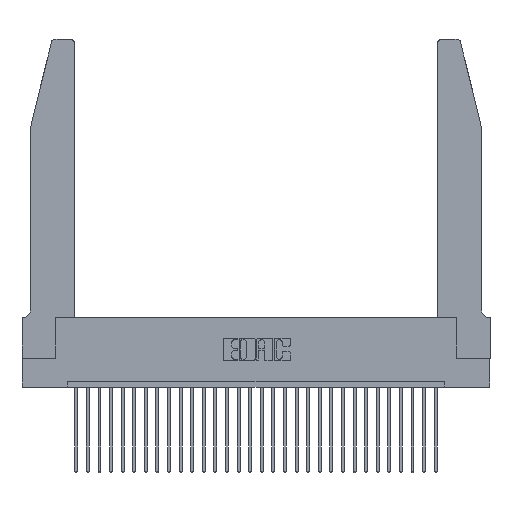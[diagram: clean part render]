
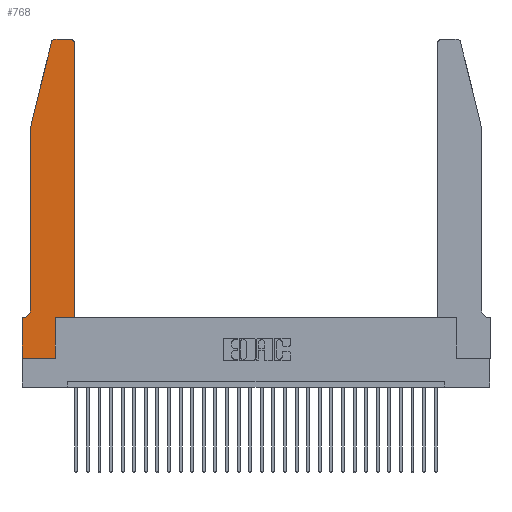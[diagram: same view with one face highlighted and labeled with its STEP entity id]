
A CAD part, top view. The second image highlights one B-rep face of the part: STEP entity #768.
In plain terms, the highlighted planar face has unit normal (0, 0, 1).
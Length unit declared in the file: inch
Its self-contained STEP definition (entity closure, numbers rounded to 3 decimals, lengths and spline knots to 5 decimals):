
#106 = CIRCLE ( 'NONE', #23955, 0.07 ) ;
#128 = CARTESIAN_POINT ( 'NONE',  ( 0.284, 2.72, 0.37 ) ) ;
#189 = CARTESIAN_POINT ( 'NONE',  ( 0., 0., 0.37 ) ) ;
#768 = ADVANCED_FACE ( 'NONE', ( #9896 ), #13526, .T. ) ;
#1057 = DIRECTION ( 'NONE',  ( -1., 0., 0. ) ) ;
#1212 = LINE ( 'NONE', #5877, #19064 ) ;
#1213 = CARTESIAN_POINT ( 'NONE',  ( 0.0755, 0.42, 0.37 ) ) ;
#1578 = EDGE_CURVE ( 'NONE', #16728, #28501, #26247, .T. ) ;
#1632 = CARTESIAN_POINT ( 'NONE',  ( 0.284, 2.75, 0.37 ) ) ;
#1847 = ORIENTED_EDGE ( 'NONE', *, *, #1578, .T. ) ;
#2159 = CARTESIAN_POINT ( 'NONE',  ( 0., 0., 0.37 ) ) ;
#2677 = EDGE_CURVE ( 'NONE', #13894, #16933, #22546, .T. ) ;
#2738 = EDGE_CURVE ( 'NONE', #5815, #26212, #29479, .T. ) ;
#3131 = DIRECTION ( 'NONE',  ( 1., 0., 0. ) ) ;
#3536 = VERTEX_POINT ( 'NONE', #14159 ) ;
#4017 = LINE ( 'NONE', #13214, #9822 ) ;
#4064 = VECTOR ( 'NONE', #15547, 39.37008 ) ;
#4070 = DIRECTION ( 'NONE',  ( 0., -1., 0. ) ) ;
#4321 = VERTEX_POINT ( 'NONE', #14307 ) ;
#5070 = CARTESIAN_POINT ( 'NONE',  ( 0.2865, 0.35, 0.37 ) ) ;
#5147 = ORIENTED_EDGE ( 'NONE', *, *, #2677, .T. ) ;
#5507 = LINE ( 'NONE', #17265, #9161 ) ;
#5815 = VERTEX_POINT ( 'NONE', #24547 ) ;
#5848 = VERTEX_POINT ( 'NONE', #1213 ) ;
#5851 = LINE ( 'NONE', #25435, #27350 ) ;
#5877 = CARTESIAN_POINT ( 'NONE',  ( 0.4505, 0.35, 0.37 ) ) ;
#5879 = AXIS2_PLACEMENT_3D ( 'NONE', #23144, #23545, #6950 ) ;
#5939 = CARTESIAN_POINT ( 'NONE',  ( 0.2865, 0., 0.37 ) ) ;
#6080 = ORIENTED_EDGE ( 'NONE', *, *, #2738, .T. ) ;
#6813 = DIRECTION ( 'NONE',  ( 1., 0., 0. ) ) ;
#6950 = DIRECTION ( 'NONE',  ( 1., 0., 0. ) ) ;
#7384 = EDGE_CURVE ( 'NONE', #10901, #3536, #1212, .T. ) ;
#7541 = ORIENTED_EDGE ( 'NONE', *, *, #28936, .T. ) ;
#8849 = EDGE_CURVE ( 'NONE', #28679, #5815, #5851, .T. ) ;
#9161 = VECTOR ( 'NONE', #3131, 39.37008 ) ;
#9822 = VECTOR ( 'NONE', #4070, 39.37008 ) ;
#9896 = FACE_OUTER_BOUND ( 'NONE', #27709, .T. ) ;
#10157 = VECTOR ( 'NONE', #23040, 39.37008 ) ;
#10209 = ORIENTED_EDGE ( 'NONE', *, *, #8849, .T. ) ;
#10570 = DIRECTION ( 'NONE',  ( 0., 1., 0. ) ) ;
#10901 = VERTEX_POINT ( 'NONE', #24233 ) ;
#10965 = ORIENTED_EDGE ( 'NONE', *, *, #25622, .T. ) ;
#10980 = CARTESIAN_POINT ( 'NONE',  ( 0.2605, 2.75, 0.37 ) ) ;
#11596 = EDGE_CURVE ( 'NONE', #5848, #28679, #106, .T. ) ;
#11744 = DIRECTION ( 'NONE',  ( 0., 0., 1. ) ) ;
#12135 = ORIENTED_EDGE ( 'NONE', *, *, #24043, .T. ) ;
#12158 = DIRECTION ( 'NONE',  ( -0.239, -0.971, 0. ) ) ;
#13214 = CARTESIAN_POINT ( 'NONE',  ( 0.0755, 2., 0.37 ) ) ;
#13310 = EDGE_CURVE ( 'NONE', #26212, #16728, #5507, .T. ) ;
#13526 = PLANE ( 'NONE',  #18339 ) ;
#13565 = DIRECTION ( 'NONE',  ( 1., 0., 0. ) ) ;
#13894 = VERTEX_POINT ( 'NONE', #26932 ) ;
#14159 = CARTESIAN_POINT ( 'NONE',  ( 0.4505, 2.72, 0.37 ) ) ;
#14307 = CARTESIAN_POINT ( 'NONE',  ( 0.0755, 2., 0.37 ) ) ;
#14521 = VECTOR ( 'NONE', #29889, 39.37008 ) ;
#15547 = DIRECTION ( 'NONE',  ( 0., 1., 0. ) ) ;
#15775 = VECTOR ( 'NONE', #12158, 39.37008 ) ;
#16141 = LINE ( 'NONE', #19104, #15775 ) ;
#16728 = VERTEX_POINT ( 'NONE', #5939 ) ;
#16933 = VERTEX_POINT ( 'NONE', #1632 ) ;
#17066 = CARTESIAN_POINT ( 'NONE',  ( 0.0055, 0.35, 0.37 ) ) ;
#17265 = CARTESIAN_POINT ( 'NONE',  ( 0., 0., 0.37 ) ) ;
#17342 = ORIENTED_EDGE ( 'NONE', *, *, #13310, .T. ) ;
#18001 = CARTESIAN_POINT ( 'NONE',  ( 0.2865, 0.35, 0.37 ) ) ;
#18339 = AXIS2_PLACEMENT_3D ( 'NONE', #25265, #20676, #6813 ) ;
#18994 = DIRECTION ( 'NONE',  ( 1., 0., 0. ) ) ;
#19064 = VECTOR ( 'NONE', #10570, 39.37008 ) ;
#19104 = CARTESIAN_POINT ( 'NONE',  ( 0.0755, 2., 0.37 ) ) ;
#19970 = ORIENTED_EDGE ( 'NONE', *, *, #11596, .T. ) ;
#20562 = DIRECTION ( 'NONE',  ( -1., 0., 0. ) ) ;
#20676 = DIRECTION ( 'NONE',  ( 0., 0., 1. ) ) ;
#20986 = LINE ( 'NONE', #27531, #26843 ) ;
#22546 = LINE ( 'NONE', #10980, #14521 ) ;
#22591 = CIRCLE ( 'NONE', #5879, 0.03 ) ;
#22804 = CARTESIAN_POINT ( 'NONE',  ( 0.25487, 2.72718, 0.37 ) ) ;
#23040 = DIRECTION ( 'NONE',  ( 0., -1., 0. ) ) ;
#23144 = CARTESIAN_POINT ( 'NONE',  ( 0.4205, 2.72, 0.37 ) ) ;
#23246 = AXIS2_PLACEMENT_3D ( 'NONE', #128, #11744, #18994 ) ;
#23545 = DIRECTION ( 'NONE',  ( 0., 0., 1. ) ) ;
#23955 = AXIS2_PLACEMENT_3D ( 'NONE', #26859, #24709, #1057 ) ;
#24043 = EDGE_CURVE ( 'NONE', #4321, #5848, #4017, .T. ) ;
#24112 = VERTEX_POINT ( 'NONE', #22804 ) ;
#24197 = ORIENTED_EDGE ( 'NONE', *, *, #26072, .T. ) ;
#24233 = CARTESIAN_POINT ( 'NONE',  ( 0.4505, 0.35, 0.37 ) ) ;
#24247 = EDGE_CURVE ( 'NONE', #3536, #13894, #22591, .T. ) ;
#24547 = CARTESIAN_POINT ( 'NONE',  ( 0., 0.35, 0.37 ) ) ;
#24709 = DIRECTION ( 'NONE',  ( 0., 0., -1. ) ) ;
#25265 = CARTESIAN_POINT ( 'NONE',  ( 0., 0.35, 0.37 ) ) ;
#25435 = CARTESIAN_POINT ( 'NONE',  ( 0.0755, 0.35, 0.37 ) ) ;
#25622 = EDGE_CURVE ( 'NONE', #16933, #24112, #29752, .T. ) ;
#25937 = ORIENTED_EDGE ( 'NONE', *, *, #24247, .T. ) ;
#26072 = EDGE_CURVE ( 'NONE', #28501, #10901, #20986, .T. ) ;
#26212 = VERTEX_POINT ( 'NONE', #189 ) ;
#26247 = LINE ( 'NONE', #18001, #4064 ) ;
#26843 = VECTOR ( 'NONE', #13565, 39.37008 ) ;
#26859 = CARTESIAN_POINT ( 'NONE',  ( 0.0055, 0.42, 0.37 ) ) ;
#26932 = CARTESIAN_POINT ( 'NONE',  ( 0.4205, 2.75, 0.37 ) ) ;
#27350 = VECTOR ( 'NONE', #20562, 39.37008 ) ;
#27531 = CARTESIAN_POINT ( 'NONE',  ( 0.4505, 0.35, 0.37 ) ) ;
#27709 = EDGE_LOOP ( 'NONE', ( #5147, #10965, #7541, #12135, #19970, #10209, #6080, #17342, #1847, #24197, #28834, #25937 ) ) ;
#28501 = VERTEX_POINT ( 'NONE', #5070 ) ;
#28679 = VERTEX_POINT ( 'NONE', #17066 ) ;
#28834 = ORIENTED_EDGE ( 'NONE', *, *, #7384, .T. ) ;
#28936 = EDGE_CURVE ( 'NONE', #24112, #4321, #16141, .T. ) ;
#29479 = LINE ( 'NONE', #2159, #10157 ) ;
#29752 = CIRCLE ( 'NONE', #23246, 0.03 ) ;
#29889 = DIRECTION ( 'NONE',  ( -1., 0., 0. ) ) ;
